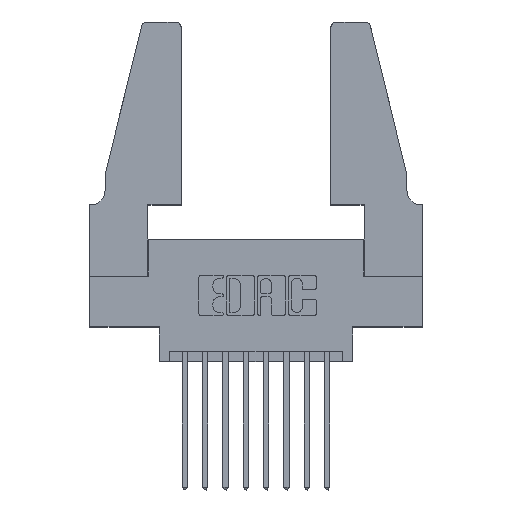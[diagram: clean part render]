
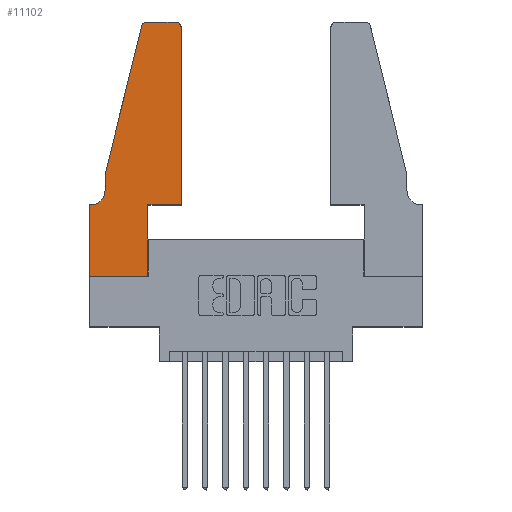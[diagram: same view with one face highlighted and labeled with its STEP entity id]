
A CAD part, top view. The second image highlights one B-rep face of the part: STEP entity #11102.
In plain terms, the highlighted planar face has unit normal (0, 0, 1).
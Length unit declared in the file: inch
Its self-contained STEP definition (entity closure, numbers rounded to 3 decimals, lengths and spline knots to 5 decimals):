
#126 = EDGE_CURVE ( 'NONE', #4426, #10890, #8945, .T. ) ;
#165 = EDGE_CURVE ( 'NONE', #5783, #1660, #324, .T. ) ;
#222 = CARTESIAN_POINT ( 'NONE',  ( 0.2865, 0.35, 0.37 ) ) ;
#324 = LINE ( 'NONE', #7445, #8320 ) ;
#431 = ORIENTED_EDGE ( 'NONE', *, *, #2710, .T. ) ;
#675 = VECTOR ( 'NONE', #9683, 39.37008 ) ;
#1060 = AXIS2_PLACEMENT_3D ( 'NONE', #4249, #11261, #5293 ) ;
#1136 = ORIENTED_EDGE ( 'NONE', *, *, #7582, .T. ) ;
#1180 = VERTEX_POINT ( 'NONE', #6019 ) ;
#1418 = EDGE_CURVE ( 'NONE', #7256, #4824, #5660, .T. ) ;
#1472 = ORIENTED_EDGE ( 'NONE', *, *, #11893, .T. ) ;
#1535 = CARTESIAN_POINT ( 'NONE',  ( 0.4205, 1.22, 0.37 ) ) ;
#1655 = DIRECTION ( 'NONE',  ( 0., 0., -1. ) ) ;
#1660 = VERTEX_POINT ( 'NONE', #3573 ) ;
#1888 = EDGE_CURVE ( 'NONE', #6032, #6521, #10358, .T. ) ;
#1965 = ORIENTED_EDGE ( 'NONE', *, *, #6237, .T. ) ;
#2135 = DIRECTION ( 'NONE',  ( 0., 0., 1. ) ) ;
#2355 = CARTESIAN_POINT ( 'NONE',  ( 0.2605, 1.25, 0.37 ) ) ;
#2467 = VECTOR ( 'NONE', #10393, 39.37008 ) ;
#2488 = EDGE_CURVE ( 'NONE', #6521, #1180, #6439, .T. ) ;
#2527 = LINE ( 'NONE', #12825, #10299 ) ;
#2665 = AXIS2_PLACEMENT_3D ( 'NONE', #1535, #8162, #2734 ) ;
#2710 = EDGE_CURVE ( 'NONE', #10329, #7256, #9564, .T. ) ;
#2734 = DIRECTION ( 'NONE',  ( 1., 0., 0. ) ) ;
#2862 = VECTOR ( 'NONE', #7561, 39.37008 ) ;
#3241 = VECTOR ( 'NONE', #7533, 39.37008 ) ;
#3294 = AXIS2_PLACEMENT_3D ( 'NONE', #7276, #2135, #9303 ) ;
#3418 = CARTESIAN_POINT ( 'NONE',  ( 0., 0., 0.37 ) ) ;
#3424 = DIRECTION ( 'NONE',  ( -1., 0., 0. ) ) ;
#3573 = CARTESIAN_POINT ( 'NONE',  ( 0.4505, 0.35, 0.37 ) ) ;
#3706 = VECTOR ( 'NONE', #3424, 39.37008 ) ;
#3843 = VERTEX_POINT ( 'NONE', #5679 ) ;
#3999 = CARTESIAN_POINT ( 'NONE',  ( 0., 0., 0.37 ) ) ;
#4249 = CARTESIAN_POINT ( 'NONE',  ( 0.284, 1.22, 0.37 ) ) ;
#4286 = ORIENTED_EDGE ( 'NONE', *, *, #8099, .T. ) ;
#4426 = VERTEX_POINT ( 'NONE', #12480 ) ;
#4618 = ORIENTED_EDGE ( 'NONE', *, *, #165, .T. ) ;
#4677 = DIRECTION ( 'NONE',  ( 0., 1., 0. ) ) ;
#4824 = VERTEX_POINT ( 'NONE', #11109 ) ;
#5293 = DIRECTION ( 'NONE',  ( 1., 0., 0. ) ) ;
#5356 = VECTOR ( 'NONE', #10709, 39.37008 ) ;
#5550 = LINE ( 'NONE', #9405, #2467 ) ;
#5660 = LINE ( 'NONE', #12506, #5356 ) ;
#5679 = CARTESIAN_POINT ( 'NONE',  ( 0.2865, 0., 0.37 ) ) ;
#5713 = ORIENTED_EDGE ( 'NONE', *, *, #6824, .T. ) ;
#5783 = VERTEX_POINT ( 'NONE', #222 ) ;
#5860 = EDGE_CURVE ( 'NONE', #1660, #6032, #9036, .T. ) ;
#6019 = CARTESIAN_POINT ( 'NONE',  ( 0.284, 1.25, 0.37 ) ) ;
#6032 = VERTEX_POINT ( 'NONE', #10925 ) ;
#6037 = ORIENTED_EDGE ( 'NONE', *, *, #1418, .T. ) ;
#6237 = EDGE_CURVE ( 'NONE', #1180, #4426, #12189, .T. ) ;
#6264 = PLANE ( 'NONE',  #3294 ) ;
#6439 = LINE ( 'NONE', #2355, #3706 ) ;
#6521 = VERTEX_POINT ( 'NONE', #11652 ) ;
#6536 = CARTESIAN_POINT ( 'NONE',  ( 0.0755, 0.5, 0.37 ) ) ;
#6824 = EDGE_CURVE ( 'NONE', #10890, #10329, #5550, .T. ) ;
#6895 = DIRECTION ( 'NONE',  ( 0., 1., 0. ) ) ;
#7131 = ORIENTED_EDGE ( 'NONE', *, *, #2488, .T. ) ;
#7256 = VERTEX_POINT ( 'NONE', #8051 ) ;
#7276 = CARTESIAN_POINT ( 'NONE',  ( 0., 0.35, 0.37 ) ) ;
#7304 = ORIENTED_EDGE ( 'NONE', *, *, #5860, .T. ) ;
#7445 = CARTESIAN_POINT ( 'NONE',  ( 0.4505, 0.35, 0.37 ) ) ;
#7458 = ORIENTED_EDGE ( 'NONE', *, *, #126, .T. ) ;
#7533 = DIRECTION ( 'NONE',  ( 1., 0., 0. ) ) ;
#7561 = DIRECTION ( 'NONE',  ( 0., -1., 0. ) ) ;
#7582 = EDGE_CURVE ( 'NONE', #4824, #8719, #13167, .T. ) ;
#7848 = CARTESIAN_POINT ( 'NONE',  ( 0.0055, 0.42, 0.37 ) ) ;
#8051 = CARTESIAN_POINT ( 'NONE',  ( 0.0055, 0.35, 0.37 ) ) ;
#8099 = EDGE_CURVE ( 'NONE', #3843, #5783, #2527, .T. ) ;
#8162 = DIRECTION ( 'NONE',  ( 0., 0., 1. ) ) ;
#8320 = VECTOR ( 'NONE', #9410, 39.37008 ) ;
#8719 = VERTEX_POINT ( 'NONE', #3999 ) ;
#8731 = VECTOR ( 'NONE', #4677, 39.37008 ) ;
#8849 = DIRECTION ( 'NONE',  ( -1., 0., 0. ) ) ;
#8945 = LINE ( 'NONE', #9669, #675 ) ;
#8993 = AXIS2_PLACEMENT_3D ( 'NONE', #7848, #1655, #8849 ) ;
#9036 = LINE ( 'NONE', #12545, #8731 ) ;
#9303 = DIRECTION ( 'NONE',  ( 1., 0., 0. ) ) ;
#9405 = CARTESIAN_POINT ( 'NONE',  ( 0.0755, 0.5, 0.37 ) ) ;
#9410 = DIRECTION ( 'NONE',  ( 1., 0., 0. ) ) ;
#9564 = CIRCLE ( 'NONE', #8993, 0.07 ) ;
#9669 = CARTESIAN_POINT ( 'NONE',  ( 0.0755, 0.5, 0.37 ) ) ;
#9683 = DIRECTION ( 'NONE',  ( -0.239, -0.971, 0. ) ) ;
#10299 = VECTOR ( 'NONE', #6895, 39.37008 ) ;
#10329 = VERTEX_POINT ( 'NONE', #10612 ) ;
#10358 = CIRCLE ( 'NONE', #2665, 0.03 ) ;
#10393 = DIRECTION ( 'NONE',  ( 0., -1., 0. ) ) ;
#10579 = ORIENTED_EDGE ( 'NONE', *, *, #1888, .T. ) ;
#10612 = CARTESIAN_POINT ( 'NONE',  ( 0.0755, 0.42, 0.37 ) ) ;
#10691 = FACE_OUTER_BOUND ( 'NONE', #11582, .T. ) ;
#10709 = DIRECTION ( 'NONE',  ( -1., 0., 0. ) ) ;
#10890 = VERTEX_POINT ( 'NONE', #6536 ) ;
#10925 = CARTESIAN_POINT ( 'NONE',  ( 0.4505, 1.22, 0.37 ) ) ;
#11102 = ADVANCED_FACE ( 'NONE', ( #10691 ), #6264, .T. ) ;
#11109 = CARTESIAN_POINT ( 'NONE',  ( 0., 0.35, 0.37 ) ) ;
#11261 = DIRECTION ( 'NONE',  ( 0., 0., 1. ) ) ;
#11277 = LINE ( 'NONE', #3418, #3241 ) ;
#11582 = EDGE_LOOP ( 'NONE', ( #7131, #1965, #7458, #5713, #431, #6037, #1136, #1472, #4286, #4618, #7304, #10579 ) ) ;
#11652 = CARTESIAN_POINT ( 'NONE',  ( 0.4205, 1.25, 0.37 ) ) ;
#11893 = EDGE_CURVE ( 'NONE', #8719, #3843, #11277, .T. ) ;
#12189 = CIRCLE ( 'NONE', #1060, 0.03 ) ;
#12423 = CARTESIAN_POINT ( 'NONE',  ( 0., 0., 0.37 ) ) ;
#12480 = CARTESIAN_POINT ( 'NONE',  ( 0.25487, 1.22718, 0.37 ) ) ;
#12506 = CARTESIAN_POINT ( 'NONE',  ( 0.0755, 0.35, 0.37 ) ) ;
#12545 = CARTESIAN_POINT ( 'NONE',  ( 0.4505, 0.35, 0.37 ) ) ;
#12825 = CARTESIAN_POINT ( 'NONE',  ( 0.2865, 0.35, 0.37 ) ) ;
#13167 = LINE ( 'NONE', #12423, #2862 ) ;
